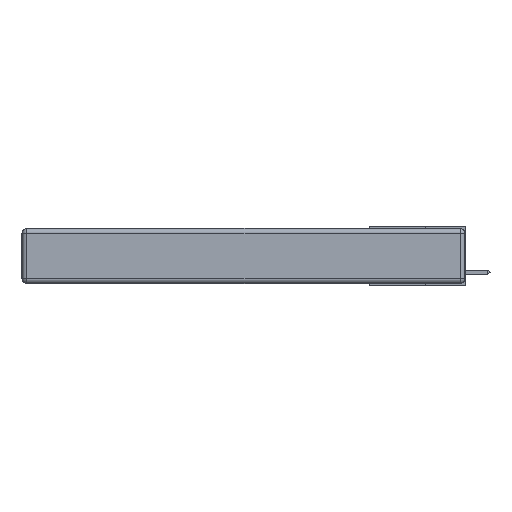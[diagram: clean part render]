
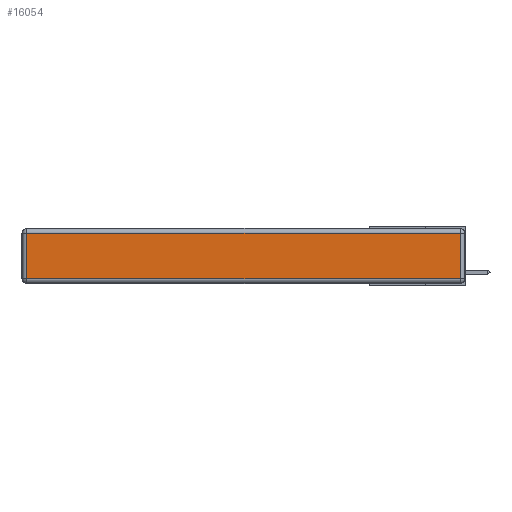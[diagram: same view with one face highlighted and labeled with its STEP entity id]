
A CAD part, left-side view. The second image highlights one B-rep face of the part: STEP entity #16054.
In plain terms, the highlighted planar face has unit normal (-1, 0, 0).
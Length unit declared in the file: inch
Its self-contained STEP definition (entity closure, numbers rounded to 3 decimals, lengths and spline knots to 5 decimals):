
#232 = VECTOR ( 'NONE', #15724, 39.37008 ) ;
#1237 = CARTESIAN_POINT ( 'NONE',  ( 0., 0., -0.343 ) ) ;
#1462 = DIRECTION ( 'NONE',  ( -1., 0., 0. ) ) ;
#1819 = EDGE_CURVE ( 'NONE', #20870, #16677, #6911, .T. ) ;
#1874 = ORIENTED_EDGE ( 'NONE', *, *, #16414, .T. ) ;
#3357 = CARTESIAN_POINT ( 'NONE',  ( 0., 0.03, -0.03 ) ) ;
#4493 = DIRECTION ( 'NONE',  ( 0., 0., 1. ) ) ;
#4609 = VECTOR ( 'NONE', #4724, 39.37008 ) ;
#4724 = DIRECTION ( 'NONE',  ( 0., 0., -1. ) ) ;
#4742 = ORIENTED_EDGE ( 'NONE', *, *, #19183, .T. ) ;
#5107 = EDGE_CURVE ( 'NONE', #18909, #14092, #14613, .T. ) ;
#5844 = FACE_OUTER_BOUND ( 'NONE', #20578, .T. ) ;
#6911 = LINE ( 'NONE', #7518, #19220 ) ;
#7518 = CARTESIAN_POINT ( 'NONE',  ( 0., 0.03, -0.343 ) ) ;
#11443 = CARTESIAN_POINT ( 'NONE',  ( 0., 2.72, -0.343 ) ) ;
#13073 = CARTESIAN_POINT ( 'NONE',  ( 0., 2.75, -0.03 ) ) ;
#13862 = LINE ( 'NONE', #16077, #232 ) ;
#14092 = VERTEX_POINT ( 'NONE', #16195 ) ;
#14613 = LINE ( 'NONE', #11443, #4609 ) ;
#14735 = PLANE ( 'NONE',  #15393 ) ;
#14983 = DIRECTION ( 'NONE',  ( 0., 1., 0. ) ) ;
#15393 = AXIS2_PLACEMENT_3D ( 'NONE', #1237, #1462, #4493 ) ;
#15721 = DIRECTION ( 'NONE',  ( 0., 0., 1. ) ) ;
#15724 = DIRECTION ( 'NONE',  ( 0., -1., 0. ) ) ;
#16054 = ADVANCED_FACE ( 'NONE', ( #5844 ), #14735, .T. ) ;
#16077 = CARTESIAN_POINT ( 'NONE',  ( 0., 0., -0.313 ) ) ;
#16195 = CARTESIAN_POINT ( 'NONE',  ( 0., 2.72, -0.313 ) ) ;
#16317 = VECTOR ( 'NONE', #14983, 39.37008 ) ;
#16414 = EDGE_CURVE ( 'NONE', #16677, #18909, #16567, .T. ) ;
#16567 = LINE ( 'NONE', #13073, #16317 ) ;
#16677 = VERTEX_POINT ( 'NONE', #3357 ) ;
#17206 = ORIENTED_EDGE ( 'NONE', *, *, #1819, .T. ) ;
#17603 = ORIENTED_EDGE ( 'NONE', *, *, #5107, .T. ) ;
#18909 = VERTEX_POINT ( 'NONE', #19666 ) ;
#19183 = EDGE_CURVE ( 'NONE', #14092, #20870, #13862, .T. ) ;
#19220 = VECTOR ( 'NONE', #15721, 39.37008 ) ;
#19666 = CARTESIAN_POINT ( 'NONE',  ( 0., 2.72, -0.03 ) ) ;
#20578 = EDGE_LOOP ( 'NONE', ( #4742, #17206, #1874, #17603 ) ) ;
#20870 = VERTEX_POINT ( 'NONE', #21123 ) ;
#21123 = CARTESIAN_POINT ( 'NONE',  ( 0., 0.03, -0.313 ) ) ;
